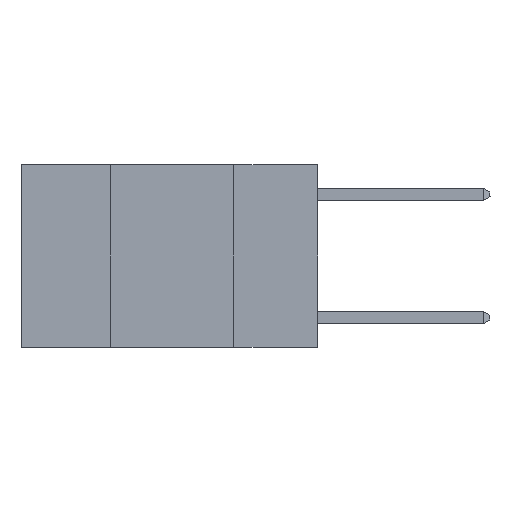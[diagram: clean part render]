
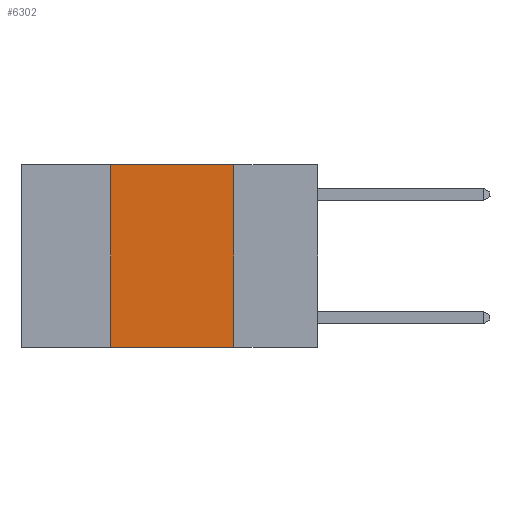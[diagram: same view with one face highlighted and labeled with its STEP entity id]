
A CAD part, left-side view. The second image highlights one B-rep face of the part: STEP entity #6302.
In plain terms, the highlighted planar face has unit normal (-1, 0, 0).
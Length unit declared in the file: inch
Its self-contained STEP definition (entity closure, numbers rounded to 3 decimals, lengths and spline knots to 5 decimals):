
#216 = CARTESIAN_POINT ( 'NONE',  ( 0., 0.17, 0. ) ) ;
#269 = VERTEX_POINT ( 'NONE', #9254 ) ;
#537 = VECTOR ( 'NONE', #3263, 39.37008 ) ;
#804 = LINE ( 'NONE', #5562, #537 ) ;
#845 = DIRECTION ( 'NONE',  ( 0., -1., 0. ) ) ;
#846 = EDGE_CURVE ( 'NONE', #5911, #3107, #7161, .T. ) ;
#894 = PLANE ( 'NONE',  #10675 ) ;
#1011 = CARTESIAN_POINT ( 'NONE',  ( 0., 0.42, -0.37 ) ) ;
#1087 = ORIENTED_EDGE ( 'NONE', *, *, #4065, .F. ) ;
#1123 = EDGE_LOOP ( 'NONE', ( #1439, #1087, #9445, #2551 ) ) ;
#1439 = ORIENTED_EDGE ( 'NONE', *, *, #846, .F. ) ;
#1800 = DIRECTION ( 'NONE',  ( 1., 0., 0. ) ) ;
#2459 = LINE ( 'NONE', #9255, #6707 ) ;
#2551 = ORIENTED_EDGE ( 'NONE', *, *, #3050, .T. ) ;
#2885 = EDGE_CURVE ( 'NONE', #6875, #269, #804, .T. ) ;
#3050 = EDGE_CURVE ( 'NONE', #6875, #3107, #4172, .T. ) ;
#3107 = VERTEX_POINT ( 'NONE', #10867 ) ;
#3263 = DIRECTION ( 'NONE',  ( 0., 0., 1. ) ) ;
#3652 = FACE_OUTER_BOUND ( 'NONE', #1123, .T. ) ;
#4065 = EDGE_CURVE ( 'NONE', #269, #5911, #2459, .T. ) ;
#4172 = LINE ( 'NONE', #10011, #6270 ) ;
#4823 = VECTOR ( 'NONE', #6633, 39.37008 ) ;
#5562 = CARTESIAN_POINT ( 'NONE',  ( 0., 0.42, 0. ) ) ;
#5911 = VERTEX_POINT ( 'NONE', #6560 ) ;
#6270 = VECTOR ( 'NONE', #845, 39.37008 ) ;
#6302 = ADVANCED_FACE ( 'NONE', ( #3652 ), #894, .F. ) ;
#6560 = CARTESIAN_POINT ( 'NONE',  ( 0., 0.17, 0. ) ) ;
#6633 = DIRECTION ( 'NONE',  ( 0., 0., -1. ) ) ;
#6707 = VECTOR ( 'NONE', #11364, 39.37008 ) ;
#6875 = VERTEX_POINT ( 'NONE', #1011 ) ;
#7161 = LINE ( 'NONE', #216, #4823 ) ;
#8064 = CARTESIAN_POINT ( 'NONE',  ( 0., 0.6, 0. ) ) ;
#8105 = DIRECTION ( 'NONE',  ( 0., 0., -1. ) ) ;
#9254 = CARTESIAN_POINT ( 'NONE',  ( 0., 0.42, 0. ) ) ;
#9255 = CARTESIAN_POINT ( 'NONE',  ( 0., 0.6, 0. ) ) ;
#9445 = ORIENTED_EDGE ( 'NONE', *, *, #2885, .F. ) ;
#10011 = CARTESIAN_POINT ( 'NONE',  ( 0., 0.6, -0.37 ) ) ;
#10675 = AXIS2_PLACEMENT_3D ( 'NONE', #8064, #1800, #8105 ) ;
#10867 = CARTESIAN_POINT ( 'NONE',  ( 0., 0.17, -0.37 ) ) ;
#11364 = DIRECTION ( 'NONE',  ( 0., -1., 0. ) ) ;
